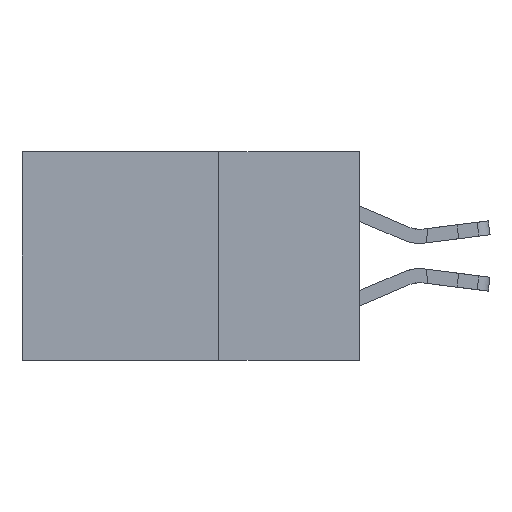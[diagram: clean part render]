
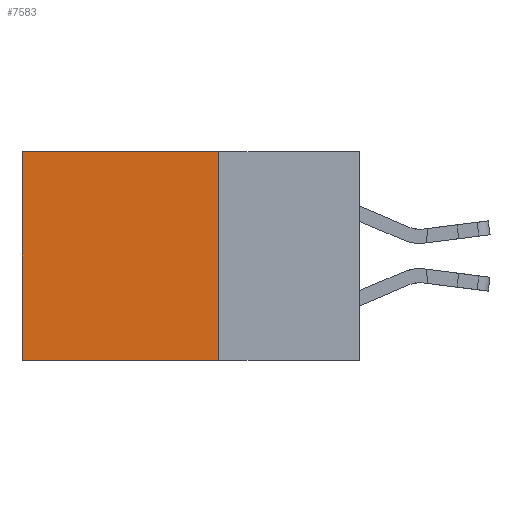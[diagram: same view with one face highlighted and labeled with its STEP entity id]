
A CAD part, left-side view. The second image highlights one B-rep face of the part: STEP entity #7583.
In plain terms, the highlighted planar face has unit normal (-1, 0, 0).
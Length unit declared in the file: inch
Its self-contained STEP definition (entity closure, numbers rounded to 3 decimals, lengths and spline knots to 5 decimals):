
#349 = CARTESIAN_POINT ( 'NONE',  ( 0.2875, 0.25, 0. ) ) ;
#690 = DIRECTION ( 'NONE',  ( 0., 1., 0. ) ) ;
#694 = CARTESIAN_POINT ( 'NONE',  ( 0.2875, 0.25, -0.37 ) ) ;
#964 = VECTOR ( 'NONE', #24392, 39.37008 ) ;
#1003 = VECTOR ( 'NONE', #21627, 39.37008 ) ;
#2196 = LINE ( 'NONE', #10416, #964 ) ;
#3353 = DIRECTION ( 'NONE',  ( 0., 0., -1. ) ) ;
#3433 = EDGE_CURVE ( 'NONE', #26171, #5464, #13753, .T. ) ;
#3626 = LINE ( 'NONE', #24044, #1003 ) ;
#4992 = CARTESIAN_POINT ( 'NONE',  ( 0.2875, 0.6, 0. ) ) ;
#5259 = FACE_OUTER_BOUND ( 'NONE', #21519, .T. ) ;
#5341 = AXIS2_PLACEMENT_3D ( 'NONE', #5391, #19364, #3353 ) ;
#5391 = CARTESIAN_POINT ( 'NONE',  ( 0.2875, 0.25, 0. ) ) ;
#5464 = VERTEX_POINT ( 'NONE', #7585 ) ;
#6377 = VERTEX_POINT ( 'NONE', #4992 ) ;
#7583 = ADVANCED_FACE ( 'NONE', ( #5259 ), #11311, .F. ) ;
#7585 = CARTESIAN_POINT ( 'NONE',  ( 0.2875, 0.6, -0.37 ) ) ;
#9367 = ORIENTED_EDGE ( 'NONE', *, *, #17541, .T. ) ;
#10416 = CARTESIAN_POINT ( 'NONE',  ( 0.2875, 0.25, 0. ) ) ;
#10674 = CARTESIAN_POINT ( 'NONE',  ( 0.2875, 0.25, 0. ) ) ;
#11311 = PLANE ( 'NONE',  #5341 ) ;
#13115 = VERTEX_POINT ( 'NONE', #349 ) ;
#13753 = LINE ( 'NONE', #17909, #26152 ) ;
#14024 = ORIENTED_EDGE ( 'NONE', *, *, #15666, .F. ) ;
#15666 = EDGE_CURVE ( 'NONE', #13115, #26171, #2196, .T. ) ;
#17541 = EDGE_CURVE ( 'NONE', #6377, #5464, #3626, .T. ) ;
#17772 = DIRECTION ( 'NONE',  ( 0., 1., 0. ) ) ;
#17909 = CARTESIAN_POINT ( 'NONE',  ( 0.2875, 0.25, -0.37 ) ) ;
#19364 = DIRECTION ( 'NONE',  ( 1., 0., 0. ) ) ;
#20545 = VECTOR ( 'NONE', #690, 39.37008 ) ;
#20582 = EDGE_CURVE ( 'NONE', #13115, #6377, #24381, .T. ) ;
#21519 = EDGE_LOOP ( 'NONE', ( #9367, #22554, #14024, #25913 ) ) ;
#21627 = DIRECTION ( 'NONE',  ( 0., 0., -1. ) ) ;
#22554 = ORIENTED_EDGE ( 'NONE', *, *, #3433, .F. ) ;
#24044 = CARTESIAN_POINT ( 'NONE',  ( 0.2875, 0.6, 0. ) ) ;
#24381 = LINE ( 'NONE', #10674, #20545 ) ;
#24392 = DIRECTION ( 'NONE',  ( 0., 0., -1. ) ) ;
#25913 = ORIENTED_EDGE ( 'NONE', *, *, #20582, .T. ) ;
#26152 = VECTOR ( 'NONE', #17772, 39.37008 ) ;
#26171 = VERTEX_POINT ( 'NONE', #694 ) ;
